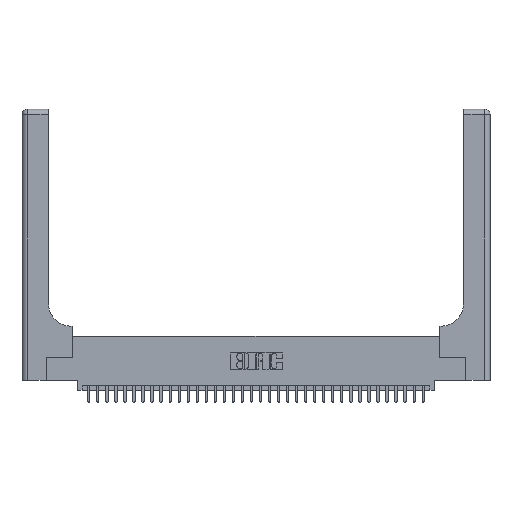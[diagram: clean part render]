
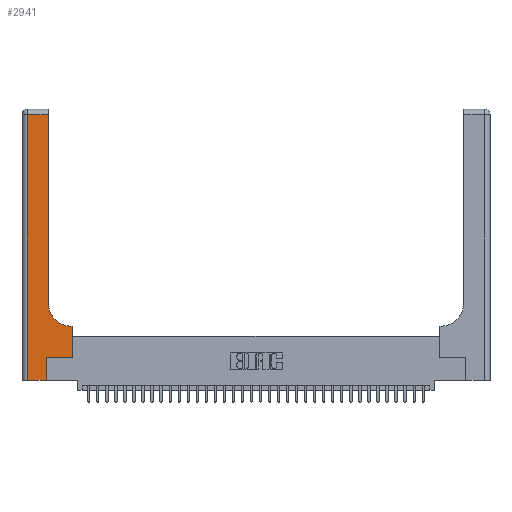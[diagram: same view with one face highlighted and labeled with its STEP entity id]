
A CAD part, top view. The second image highlights one B-rep face of the part: STEP entity #2941.
In plain terms, the highlighted planar face has unit normal (0, 0, 1).
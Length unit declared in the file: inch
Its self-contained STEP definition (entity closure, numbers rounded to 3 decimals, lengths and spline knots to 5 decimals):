
#270 = LINE ( 'NONE', #23071, #27470 ) ;
#988 = LINE ( 'NONE', #3004, #1414 ) ;
#1414 = VECTOR ( 'NONE', #35679, 39.37008 ) ;
#1543 = CARTESIAN_POINT ( 'NONE',  ( 0.06, 2.94, 0.37 ) ) ;
#2114 = AXIS2_PLACEMENT_3D ( 'NONE', #35575, #8474, #7758 ) ;
#2850 = EDGE_CURVE ( 'NONE', #33637, #27226, #270, .T. ) ;
#2941 = ADVANCED_FACE ( 'NONE', ( #27882 ), #17329, .F. ) ;
#3004 = CARTESIAN_POINT ( 'NONE',  ( 0., 0., 0.37 ) ) ;
#3032 = CARTESIAN_POINT ( 'NONE',  ( 0.2915, 0.85, 0.37 ) ) ;
#3559 = ORIENTED_EDGE ( 'NONE', *, *, #16862, .T. ) ;
#4324 = CARTESIAN_POINT ( 'NONE',  ( 0.06, 3., 0.37 ) ) ;
#4858 = ORIENTED_EDGE ( 'NONE', *, *, #29030, .T. ) ;
#5010 = CARTESIAN_POINT ( 'NONE',  ( 0.269, 0.25, 0.37 ) ) ;
#6032 = EDGE_CURVE ( 'NONE', #26401, #24218, #20197, .T. ) ;
#6101 = VECTOR ( 'NONE', #23681, 39.37008 ) ;
#6420 = VECTOR ( 'NONE', #20975, 39.37008 ) ;
#7391 = DIRECTION ( 'NONE',  ( 0., 0., -1. ) ) ;
#7758 = DIRECTION ( 'NONE',  ( -1., 0., 0. ) ) ;
#8005 = CARTESIAN_POINT ( 'NONE',  ( 0.5585, 0.25, 0.37 ) ) ;
#8248 = ORIENTED_EDGE ( 'NONE', *, *, #19838, .T. ) ;
#8474 = DIRECTION ( 'NONE',  ( 0., 0., -1. ) ) ;
#8501 = EDGE_CURVE ( 'NONE', #11468, #26401, #23898, .T. ) ;
#9308 = CARTESIAN_POINT ( 'NONE',  ( 0.5415, 0.85, 0.37 ) ) ;
#9741 = VECTOR ( 'NONE', #16375, 39.37008 ) ;
#9992 = ORIENTED_EDGE ( 'NONE', *, *, #11913, .T. ) ;
#10937 = VERTEX_POINT ( 'NONE', #1543 ) ;
#11468 = VERTEX_POINT ( 'NONE', #13277 ) ;
#11913 = EDGE_CURVE ( 'NONE', #18742, #11468, #988, .T. ) ;
#12089 = ORIENTED_EDGE ( 'NONE', *, *, #8501, .T. ) ;
#12811 = CARTESIAN_POINT ( 'NONE',  ( 0.5585, 0.25, 0.37 ) ) ;
#12820 = CARTESIAN_POINT ( 'NONE',  ( 0.2915, 0.6, 0.37 ) ) ;
#13232 = CIRCLE ( 'NONE', #26811, 0.25 ) ;
#13277 = CARTESIAN_POINT ( 'NONE',  ( 0.269, 0., 0.37 ) ) ;
#13471 = EDGE_CURVE ( 'NONE', #10937, #18742, #22440, .T. ) ;
#16375 = DIRECTION ( 'NONE',  ( 0., 1., 0. ) ) ;
#16862 = EDGE_CURVE ( 'NONE', #23303, #33637, #13232, .T. ) ;
#17329 = PLANE ( 'NONE',  #2114 ) ;
#17996 = ORIENTED_EDGE ( 'NONE', *, *, #18251, .T. ) ;
#18251 = EDGE_CURVE ( 'NONE', #24218, #18824, #30859, .T. ) ;
#18469 = DIRECTION ( 'NONE',  ( 1., 0., 0. ) ) ;
#18742 = VERTEX_POINT ( 'NONE', #35670 ) ;
#18824 = VERTEX_POINT ( 'NONE', #26993 ) ;
#19838 = EDGE_CURVE ( 'NONE', #27226, #10937, #22506, .T. ) ;
#20197 = LINE ( 'NONE', #5010, #27525 ) ;
#20463 = CARTESIAN_POINT ( 'NONE',  ( 0.5415, 0.6, 0.37 ) ) ;
#20975 = DIRECTION ( 'NONE',  ( -1., 0., 0. ) ) ;
#21748 = CARTESIAN_POINT ( 'NONE',  ( 0.269, 0., 0.37 ) ) ;
#22440 = LINE ( 'NONE', #4324, #6101 ) ;
#22506 = LINE ( 'NONE', #34728, #25111 ) ;
#23071 = CARTESIAN_POINT ( 'NONE',  ( 0.2915, 3., 0.37 ) ) ;
#23303 = VERTEX_POINT ( 'NONE', #20463 ) ;
#23681 = DIRECTION ( 'NONE',  ( 0., -1., 0. ) ) ;
#23898 = LINE ( 'NONE', #21748, #9741 ) ;
#24218 = VERTEX_POINT ( 'NONE', #12811 ) ;
#25111 = VECTOR ( 'NONE', #34849, 39.37008 ) ;
#25274 = CARTESIAN_POINT ( 'NONE',  ( 0.269, 0.25, 0.37 ) ) ;
#25617 = VECTOR ( 'NONE', #30006, 39.37008 ) ;
#26246 = LINE ( 'NONE', #12820, #6420 ) ;
#26401 = VERTEX_POINT ( 'NONE', #25274 ) ;
#26456 = CARTESIAN_POINT ( 'NONE',  ( 0.2915, 2.94, 0.37 ) ) ;
#26811 = AXIS2_PLACEMENT_3D ( 'NONE', #9308, #7391, #18469 ) ;
#26993 = CARTESIAN_POINT ( 'NONE',  ( 0.5585, 0.6, 0.37 ) ) ;
#27226 = VERTEX_POINT ( 'NONE', #26456 ) ;
#27363 = DIRECTION ( 'NONE',  ( 1., 0., 0. ) ) ;
#27470 = VECTOR ( 'NONE', #35690, 39.37008 ) ;
#27525 = VECTOR ( 'NONE', #27363, 39.37008 ) ;
#27610 = EDGE_LOOP ( 'NONE', ( #34482, #8248, #33377, #9992, #12089, #34770, #17996, #4858, #3559 ) ) ;
#27882 = FACE_OUTER_BOUND ( 'NONE', #27610, .T. ) ;
#29030 = EDGE_CURVE ( 'NONE', #18824, #23303, #26246, .T. ) ;
#30006 = DIRECTION ( 'NONE',  ( 0., 1., 0. ) ) ;
#30859 = LINE ( 'NONE', #8005, #25617 ) ;
#33377 = ORIENTED_EDGE ( 'NONE', *, *, #13471, .T. ) ;
#33637 = VERTEX_POINT ( 'NONE', #3032 ) ;
#34482 = ORIENTED_EDGE ( 'NONE', *, *, #2850, .T. ) ;
#34728 = CARTESIAN_POINT ( 'NONE',  ( 0., 2.94, 0.37 ) ) ;
#34770 = ORIENTED_EDGE ( 'NONE', *, *, #6032, .T. ) ;
#34849 = DIRECTION ( 'NONE',  ( -1., 0., 0. ) ) ;
#35575 = CARTESIAN_POINT ( 'NONE',  ( 0., 3., 0.37 ) ) ;
#35670 = CARTESIAN_POINT ( 'NONE',  ( 0.06, 0., 0.37 ) ) ;
#35679 = DIRECTION ( 'NONE',  ( 1., 0., 0. ) ) ;
#35690 = DIRECTION ( 'NONE',  ( 0., 1., 0. ) ) ;
